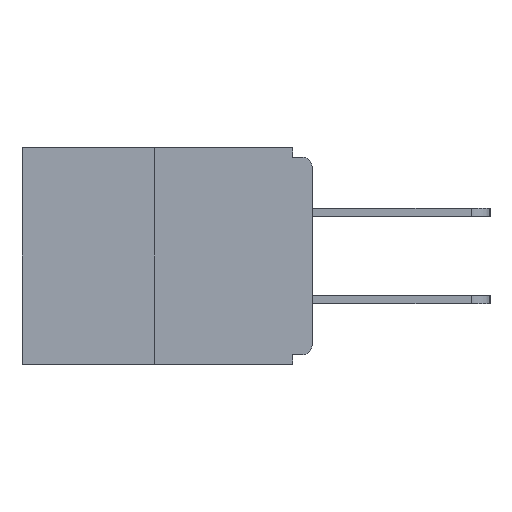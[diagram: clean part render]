
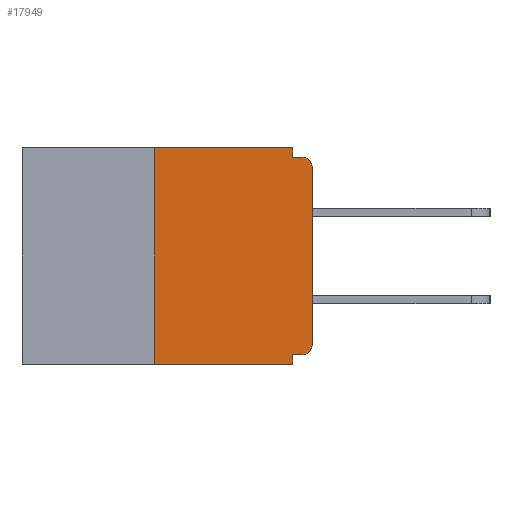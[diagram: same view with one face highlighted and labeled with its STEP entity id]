
A CAD part, left-side view. The second image highlights one B-rep face of the part: STEP entity #17949.
In plain terms, the highlighted planar face has unit normal (-1, 0, 0).
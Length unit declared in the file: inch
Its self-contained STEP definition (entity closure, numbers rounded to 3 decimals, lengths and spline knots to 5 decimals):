
#26 = VERTEX_POINT ( 'NONE', #7010 ) ;
#814 = EDGE_CURVE ( 'NONE', #21787, #4133, #10088, .T. ) ;
#968 = VERTEX_POINT ( 'NONE', #3509 ) ;
#1082 = EDGE_CURVE ( 'NONE', #15103, #968, #20616, .T. ) ;
#1093 = LINE ( 'NONE', #6911, #19050 ) ;
#1564 = DIRECTION ( 'NONE',  ( 1., 0., 0. ) ) ;
#1682 = CARTESIAN_POINT ( 'NONE',  ( 0., 0.46, 0. ) ) ;
#1696 = DIRECTION ( 'NONE',  ( 0., 0., -1. ) ) ;
#1746 = VECTOR ( 'NONE', #9190, 39.37008 ) ;
#1778 = VECTOR ( 'NONE', #8389, 39.37008 ) ;
#3018 = CARTESIAN_POINT ( 'NONE',  ( 0., 0., -0.015 ) ) ;
#3093 = LINE ( 'NONE', #1682, #13125 ) ;
#3430 = CARTESIAN_POINT ( 'NONE',  ( 0., 0., 0. ) ) ;
#3473 = LINE ( 'NONE', #6969, #1746 ) ;
#3509 = CARTESIAN_POINT ( 'NONE',  ( 0., 0.015, -0.015 ) ) ;
#3631 = LINE ( 'NONE', #9211, #9690 ) ;
#3655 = DIRECTION ( 'NONE',  ( 0., 1., 0. ) ) ;
#3720 = EDGE_CURVE ( 'NONE', #21787, #21267, #3631, .T. ) ;
#4004 = AXIS2_PLACEMENT_3D ( 'NONE', #20386, #8366, #16342 ) ;
#4133 = VERTEX_POINT ( 'NONE', #6445 ) ;
#4564 = AXIS2_PLACEMENT_3D ( 'NONE', #17943, #1564, #1696 ) ;
#5166 = DIRECTION ( 'NONE',  ( 0., -1., 0. ) ) ;
#5715 = ORIENTED_EDGE ( 'NONE', *, *, #19565, .F. ) ;
#5907 = EDGE_CURVE ( 'NONE', #23861, #20860, #13421, .T. ) ;
#6132 = ORIENTED_EDGE ( 'NONE', *, *, #22077, .F. ) ;
#6445 = CARTESIAN_POINT ( 'NONE',  ( 0., 0.25, 0. ) ) ;
#6911 = CARTESIAN_POINT ( 'NONE',  ( 0., 0.031, -0.343 ) ) ;
#6969 = CARTESIAN_POINT ( 'NONE',  ( 0., 0.031, 0. ) ) ;
#7010 = CARTESIAN_POINT ( 'NONE',  ( 0., 0.031, 0. ) ) ;
#7726 = EDGE_CURVE ( 'NONE', #21824, #10053, #23496, .T. ) ;
#8207 = ORIENTED_EDGE ( 'NONE', *, *, #12118, .F. ) ;
#8366 = DIRECTION ( 'NONE',  ( -1., 0., 0. ) ) ;
#8389 = DIRECTION ( 'NONE',  ( 0., 0., 1. ) ) ;
#8639 = ORIENTED_EDGE ( 'NONE', *, *, #3720, .T. ) ;
#8898 = VECTOR ( 'NONE', #15007, 39.37008 ) ;
#8974 = CIRCLE ( 'NONE', #4004, 0.015 ) ;
#9190 = DIRECTION ( 'NONE',  ( 0., 0., -1. ) ) ;
#9211 = CARTESIAN_POINT ( 'NONE',  ( 0., 0.46, -0.343 ) ) ;
#9506 = CARTESIAN_POINT ( 'NONE',  ( 0., 0.031, -0.015 ) ) ;
#9690 = VECTOR ( 'NONE', #11568, 39.37008 ) ;
#10053 = VERTEX_POINT ( 'NONE', #19639 ) ;
#10088 = LINE ( 'NONE', #24045, #1778 ) ;
#11440 = PLANE ( 'NONE',  #4564 ) ;
#11568 = DIRECTION ( 'NONE',  ( 0., -1., 0. ) ) ;
#12118 = EDGE_CURVE ( 'NONE', #20860, #21267, #1093, .T. ) ;
#12313 = EDGE_LOOP ( 'NONE', ( #6132, #15746, #8639, #8207, #13480, #16990, #15225, #25097, #20013, #5715 ) ) ;
#12419 = AXIS2_PLACEMENT_3D ( 'NONE', #23964, #19686, #17851 ) ;
#13125 = VECTOR ( 'NONE', #5166, 39.37008 ) ;
#13421 = LINE ( 'NONE', #25305, #25136 ) ;
#13480 = ORIENTED_EDGE ( 'NONE', *, *, #5907, .F. ) ;
#13923 = CARTESIAN_POINT ( 'NONE',  ( 0., 0., -0.313 ) ) ;
#15007 = DIRECTION ( 'NONE',  ( 0., -1., 0. ) ) ;
#15103 = VERTEX_POINT ( 'NONE', #9506 ) ;
#15225 = ORIENTED_EDGE ( 'NONE', *, *, #7726, .T. ) ;
#15746 = ORIENTED_EDGE ( 'NONE', *, *, #814, .F. ) ;
#16342 = DIRECTION ( 'NONE',  ( 0., 0., -1. ) ) ;
#16990 = ORIENTED_EDGE ( 'NONE', *, *, #22836, .T. ) ;
#17508 = DIRECTION ( 'NONE',  ( 0., 0., 1. ) ) ;
#17851 = DIRECTION ( 'NONE',  ( 0., 0., -1. ) ) ;
#17943 = CARTESIAN_POINT ( 'NONE',  ( 0., 0.46, 0. ) ) ;
#17949 = ADVANCED_FACE ( 'NONE', ( #23820 ), #11440, .F. ) ;
#18807 = DIRECTION ( 'NONE',  ( 0., 0., -1. ) ) ;
#18885 = VECTOR ( 'NONE', #17508, 39.37008 ) ;
#19050 = VECTOR ( 'NONE', #18807, 39.37008 ) ;
#19565 = EDGE_CURVE ( 'NONE', #26, #15103, #3473, .T. ) ;
#19639 = CARTESIAN_POINT ( 'NONE',  ( 0., 0., -0.03 ) ) ;
#19686 = DIRECTION ( 'NONE',  ( -1., 0., 0. ) ) ;
#19999 = CARTESIAN_POINT ( 'NONE',  ( 0., 0.015, -0.328 ) ) ;
#20013 = ORIENTED_EDGE ( 'NONE', *, *, #1082, .F. ) ;
#20386 = CARTESIAN_POINT ( 'NONE',  ( 0., 0.015, -0.313 ) ) ;
#20616 = LINE ( 'NONE', #3018, #8898 ) ;
#20860 = VERTEX_POINT ( 'NONE', #21331 ) ;
#21267 = VERTEX_POINT ( 'NONE', #25229 ) ;
#21331 = CARTESIAN_POINT ( 'NONE',  ( 0., 0.031, -0.328 ) ) ;
#21787 = VERTEX_POINT ( 'NONE', #23834 ) ;
#21824 = VERTEX_POINT ( 'NONE', #13923 ) ;
#22077 = EDGE_CURVE ( 'NONE', #4133, #26, #3093, .T. ) ;
#22836 = EDGE_CURVE ( 'NONE', #23861, #21824, #8974, .T. ) ;
#23496 = LINE ( 'NONE', #3430, #18885 ) ;
#23820 = FACE_OUTER_BOUND ( 'NONE', #12313, .T. ) ;
#23834 = CARTESIAN_POINT ( 'NONE',  ( 0., 0.25, -0.343 ) ) ;
#23861 = VERTEX_POINT ( 'NONE', #19999 ) ;
#23964 = CARTESIAN_POINT ( 'NONE',  ( 0., 0.015, -0.03 ) ) ;
#24045 = CARTESIAN_POINT ( 'NONE',  ( 0., 0.25, 0. ) ) ;
#24671 = EDGE_CURVE ( 'NONE', #10053, #968, #25332, .T. ) ;
#25097 = ORIENTED_EDGE ( 'NONE', *, *, #24671, .T. ) ;
#25136 = VECTOR ( 'NONE', #3655, 39.37008 ) ;
#25229 = CARTESIAN_POINT ( 'NONE',  ( 0., 0.031, -0.343 ) ) ;
#25305 = CARTESIAN_POINT ( 'NONE',  ( 0., 0., -0.328 ) ) ;
#25332 = CIRCLE ( 'NONE', #12419, 0.015 ) ;
